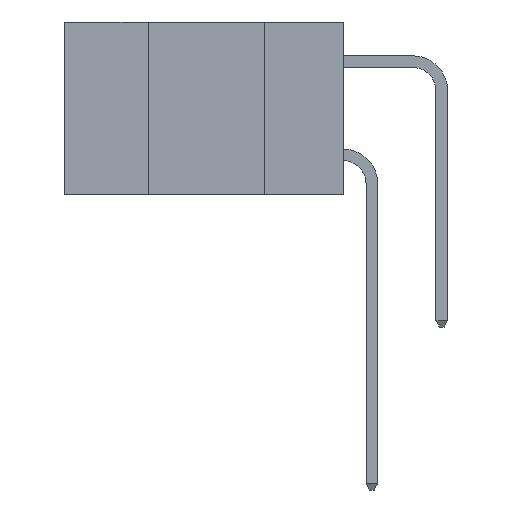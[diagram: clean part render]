
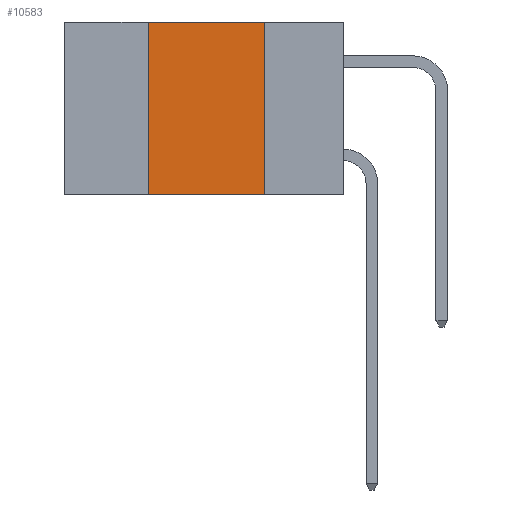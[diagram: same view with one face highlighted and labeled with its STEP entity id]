
A CAD part, left-side view. The second image highlights one B-rep face of the part: STEP entity #10583.
In plain terms, the highlighted planar face has unit normal (-1, 0, 0).
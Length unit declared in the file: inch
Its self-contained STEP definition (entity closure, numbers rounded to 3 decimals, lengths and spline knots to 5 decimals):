
#379 = VECTOR ( 'NONE', #5873, 39.37008 ) ;
#748 = VECTOR ( 'NONE', #7521, 39.37008 ) ;
#758 = CARTESIAN_POINT ( 'NONE',  ( 0., 0.6, -0.37 ) ) ;
#911 = EDGE_LOOP ( 'NONE', ( #5778, #14420, #6598, #8739 ) ) ;
#1397 = FACE_OUTER_BOUND ( 'NONE', #911, .T. ) ;
#1751 = AXIS2_PLACEMENT_3D ( 'NONE', #4167, #5456, #14254 ) ;
#2486 = CARTESIAN_POINT ( 'NONE',  ( 0., 0.42, -0.37 ) ) ;
#3369 = VECTOR ( 'NONE', #11606, 39.37008 ) ;
#3638 = EDGE_CURVE ( 'NONE', #3819, #12072, #14173, .T. ) ;
#3734 = LINE ( 'NONE', #758, #379 ) ;
#3819 = VERTEX_POINT ( 'NONE', #4646 ) ;
#3999 = CARTESIAN_POINT ( 'NONE',  ( 0., 0.42, -0.37 ) ) ;
#4095 = EDGE_CURVE ( 'NONE', #12925, #3819, #4100, .T. ) ;
#4100 = LINE ( 'NONE', #7093, #7876 ) ;
#4167 = CARTESIAN_POINT ( 'NONE',  ( 0., 0.6, 0. ) ) ;
#4646 = CARTESIAN_POINT ( 'NONE',  ( 0., 0.17, 0. ) ) ;
#5456 = DIRECTION ( 'NONE',  ( 1., 0., 0. ) ) ;
#5778 = ORIENTED_EDGE ( 'NONE', *, *, #3638, .F. ) ;
#5873 = DIRECTION ( 'NONE',  ( 0., -1., 0. ) ) ;
#6304 = DIRECTION ( 'NONE',  ( 0., -1., 0. ) ) ;
#6598 = ORIENTED_EDGE ( 'NONE', *, *, #10510, .F. ) ;
#7093 = CARTESIAN_POINT ( 'NONE',  ( 0., 0.6, 0. ) ) ;
#7521 = DIRECTION ( 'NONE',  ( 0., 0., -1. ) ) ;
#7730 = CARTESIAN_POINT ( 'NONE',  ( 0., 0.17, -0.37 ) ) ;
#7876 = VECTOR ( 'NONE', #6304, 39.37008 ) ;
#8739 = ORIENTED_EDGE ( 'NONE', *, *, #12111, .T. ) ;
#9298 = VERTEX_POINT ( 'NONE', #2486 ) ;
#10510 = EDGE_CURVE ( 'NONE', #9298, #12925, #11888, .T. ) ;
#10583 = ADVANCED_FACE ( 'NONE', ( #1397 ), #13032, .F. ) ;
#11575 = CARTESIAN_POINT ( 'NONE',  ( 0., 0.42, 0. ) ) ;
#11606 = DIRECTION ( 'NONE',  ( 0., 0., 1. ) ) ;
#11888 = LINE ( 'NONE', #3999, #3369 ) ;
#12072 = VERTEX_POINT ( 'NONE', #14538 ) ;
#12111 = EDGE_CURVE ( 'NONE', #9298, #12072, #3734, .T. ) ;
#12925 = VERTEX_POINT ( 'NONE', #11575 ) ;
#13032 = PLANE ( 'NONE',  #1751 ) ;
#14173 = LINE ( 'NONE', #7730, #748 ) ;
#14254 = DIRECTION ( 'NONE',  ( 0., 0., -1. ) ) ;
#14420 = ORIENTED_EDGE ( 'NONE', *, *, #4095, .F. ) ;
#14538 = CARTESIAN_POINT ( 'NONE',  ( 0., 0.17, -0.37 ) ) ;
